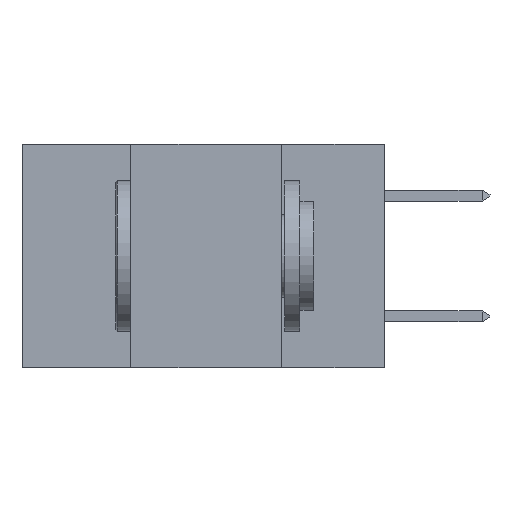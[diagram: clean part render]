
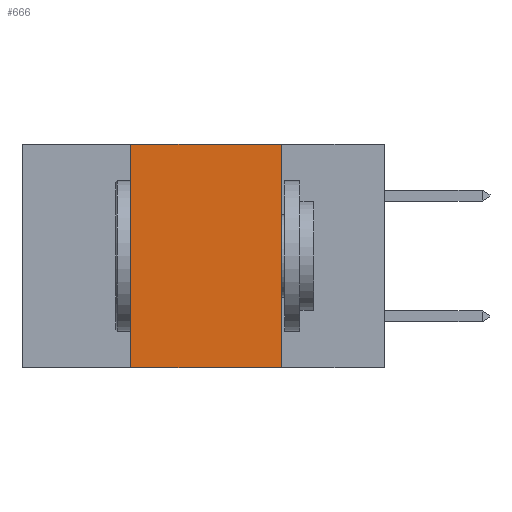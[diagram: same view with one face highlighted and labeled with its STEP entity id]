
A CAD part, left-side view. The second image highlights one B-rep face of the part: STEP entity #666.
In plain terms, the highlighted planar face has unit normal (-1, 0, 0).
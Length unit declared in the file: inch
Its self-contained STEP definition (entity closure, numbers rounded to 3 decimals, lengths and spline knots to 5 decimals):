
#62 = DIRECTION ( 'NONE',  ( 0., -1., 0. ) ) ;
#213 = LINE ( 'NONE', #13659, #5490 ) ;
#666 = ADVANCED_FACE ( 'NONE', ( #2665 ), #3120, .F. ) ;
#720 = EDGE_CURVE ( 'NONE', #1443, #4059, #5286, .T. ) ;
#1366 = VERTEX_POINT ( 'NONE', #2136 ) ;
#1443 = VERTEX_POINT ( 'NONE', #8722 ) ;
#1822 = CARTESIAN_POINT ( 'NONE',  ( 0., 0.6, -0.37 ) ) ;
#2136 = CARTESIAN_POINT ( 'NONE',  ( 0., 0.42, 0. ) ) ;
#2665 = FACE_OUTER_BOUND ( 'NONE', #7088, .T. ) ;
#2801 = CARTESIAN_POINT ( 'NONE',  ( 0., 0.42, -0.37 ) ) ;
#2924 = DIRECTION ( 'NONE',  ( 0., -1., 0. ) ) ;
#3120 = PLANE ( 'NONE',  #4899 ) ;
#3276 = CARTESIAN_POINT ( 'NONE',  ( 0., 0.17, -0.37 ) ) ;
#3413 = CARTESIAN_POINT ( 'NONE',  ( 0., 0.17, 0. ) ) ;
#4059 = VERTEX_POINT ( 'NONE', #3276 ) ;
#4768 = EDGE_CURVE ( 'NONE', #7647, #1366, #213, .T. ) ;
#4899 = AXIS2_PLACEMENT_3D ( 'NONE', #10915, #9778, #9316 ) ;
#5107 = LINE ( 'NONE', #9014, #10669 ) ;
#5286 = LINE ( 'NONE', #3413, #11887 ) ;
#5490 = VECTOR ( 'NONE', #14247, 39.37008 ) ;
#5510 = ORIENTED_EDGE ( 'NONE', *, *, #6334, .T. ) ;
#5814 = LINE ( 'NONE', #1822, #11387 ) ;
#6334 = EDGE_CURVE ( 'NONE', #7647, #4059, #5814, .T. ) ;
#6859 = DIRECTION ( 'NONE',  ( 0., 0., -1. ) ) ;
#7088 = EDGE_LOOP ( 'NONE', ( #10054, #13281, #13621, #5510 ) ) ;
#7647 = VERTEX_POINT ( 'NONE', #2801 ) ;
#8397 = EDGE_CURVE ( 'NONE', #1366, #1443, #5107, .T. ) ;
#8722 = CARTESIAN_POINT ( 'NONE',  ( 0., 0.17, 0. ) ) ;
#9014 = CARTESIAN_POINT ( 'NONE',  ( 0., 0.6, 0. ) ) ;
#9316 = DIRECTION ( 'NONE',  ( 0., 0., -1. ) ) ;
#9778 = DIRECTION ( 'NONE',  ( 1., 0., 0. ) ) ;
#10054 = ORIENTED_EDGE ( 'NONE', *, *, #720, .F. ) ;
#10669 = VECTOR ( 'NONE', #62, 39.37008 ) ;
#10915 = CARTESIAN_POINT ( 'NONE',  ( 0., 0.6, 0. ) ) ;
#11387 = VECTOR ( 'NONE', #2924, 39.37008 ) ;
#11887 = VECTOR ( 'NONE', #6859, 39.37008 ) ;
#13281 = ORIENTED_EDGE ( 'NONE', *, *, #8397, .F. ) ;
#13621 = ORIENTED_EDGE ( 'NONE', *, *, #4768, .F. ) ;
#13659 = CARTESIAN_POINT ( 'NONE',  ( 0., 0.42, 0. ) ) ;
#14247 = DIRECTION ( 'NONE',  ( 0., 0., 1. ) ) ;
